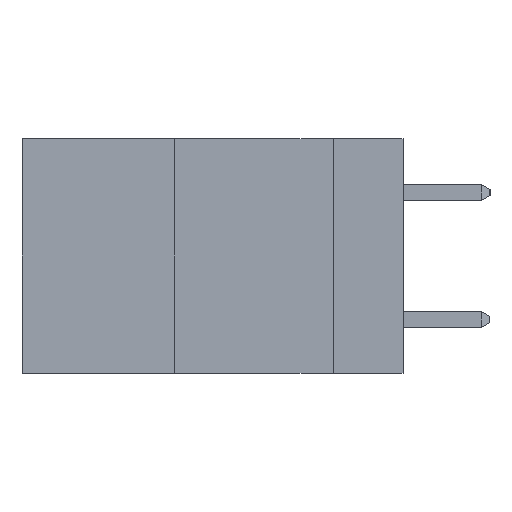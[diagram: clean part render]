
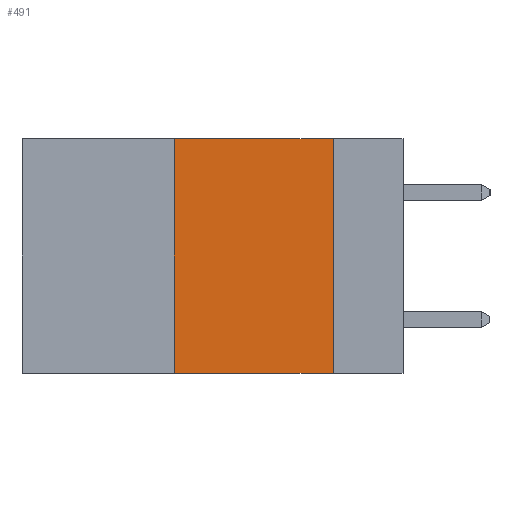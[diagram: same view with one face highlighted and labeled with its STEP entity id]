
A CAD part, left-side view. The second image highlights one B-rep face of the part: STEP entity #491.
In plain terms, the highlighted planar face has unit normal (-1, 0, 0).
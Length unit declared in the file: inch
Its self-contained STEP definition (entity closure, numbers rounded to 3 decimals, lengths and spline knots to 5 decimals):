
#68 = VECTOR ( 'NONE', #825, 39.37008 ) ;
#221 = VERTEX_POINT ( 'NONE', #890 ) ;
#350 = ORIENTED_EDGE ( 'NONE', *, *, #613, .T. ) ;
#491 = ADVANCED_FACE ( 'NONE', ( #6670 ), #3506, .F. ) ;
#613 = EDGE_CURVE ( 'NONE', #221, #9625, #7076, .T. ) ;
#825 = DIRECTION ( 'NONE',  ( 0., -1., 0. ) ) ;
#890 = CARTESIAN_POINT ( 'NONE',  ( 0., 0.36, -0.37 ) ) ;
#1199 = EDGE_CURVE ( 'NONE', #221, #3394, #5819, .T. ) ;
#1262 = LINE ( 'NONE', #9466, #1528 ) ;
#1392 = DIRECTION ( 'NONE',  ( 1., 0., 0. ) ) ;
#1528 = VECTOR ( 'NONE', #6396, 39.37008 ) ;
#2752 = EDGE_CURVE ( 'NONE', #3394, #7671, #3537, .T. ) ;
#3394 = VERTEX_POINT ( 'NONE', #5705 ) ;
#3466 = CARTESIAN_POINT ( 'NONE',  ( 0., 0.36, 0. ) ) ;
#3506 = PLANE ( 'NONE',  #7452 ) ;
#3537 = LINE ( 'NONE', #4452, #3982 ) ;
#3982 = VECTOR ( 'NONE', #9769, 39.37008 ) ;
#4289 = ORIENTED_EDGE ( 'NONE', *, *, #1199, .F. ) ;
#4452 = CARTESIAN_POINT ( 'NONE',  ( 0., 0.6, 0. ) ) ;
#4460 = ORIENTED_EDGE ( 'NONE', *, *, #2752, .F. ) ;
#5688 = VECTOR ( 'NONE', #5768, 39.37008 ) ;
#5705 = CARTESIAN_POINT ( 'NONE',  ( 0., 0.36, 0. ) ) ;
#5768 = DIRECTION ( 'NONE',  ( 0., 0., 1. ) ) ;
#5819 = LINE ( 'NONE', #3466, #5688 ) ;
#5892 = CARTESIAN_POINT ( 'NONE',  ( 0., 0.11, 0. ) ) ;
#5906 = CARTESIAN_POINT ( 'NONE',  ( 0., 0.6, 0. ) ) ;
#6396 = DIRECTION ( 'NONE',  ( 0., 0., -1. ) ) ;
#6617 = DIRECTION ( 'NONE',  ( 0., 0., -1. ) ) ;
#6670 = FACE_OUTER_BOUND ( 'NONE', #9996, .T. ) ;
#6904 = ORIENTED_EDGE ( 'NONE', *, *, #8434, .F. ) ;
#7076 = LINE ( 'NONE', #8622, #68 ) ;
#7452 = AXIS2_PLACEMENT_3D ( 'NONE', #5906, #1392, #6617 ) ;
#7671 = VERTEX_POINT ( 'NONE', #5892 ) ;
#8434 = EDGE_CURVE ( 'NONE', #7671, #9625, #1262, .T. ) ;
#8554 = CARTESIAN_POINT ( 'NONE',  ( 0., 0.11, -0.37 ) ) ;
#8622 = CARTESIAN_POINT ( 'NONE',  ( 0., 0.6, -0.37 ) ) ;
#9466 = CARTESIAN_POINT ( 'NONE',  ( 0., 0.11, 0. ) ) ;
#9625 = VERTEX_POINT ( 'NONE', #8554 ) ;
#9769 = DIRECTION ( 'NONE',  ( 0., -1., 0. ) ) ;
#9996 = EDGE_LOOP ( 'NONE', ( #6904, #4460, #4289, #350 ) ) ;
